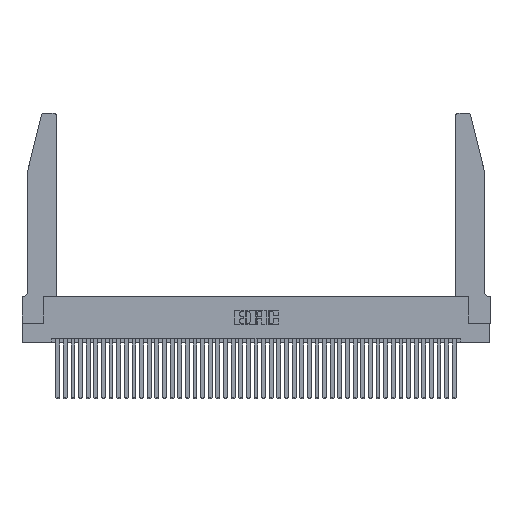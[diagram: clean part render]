
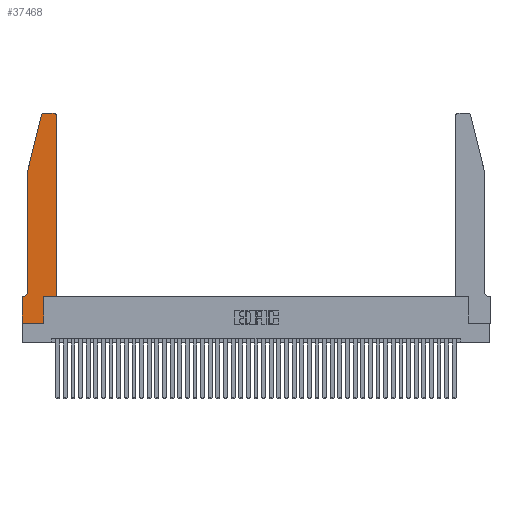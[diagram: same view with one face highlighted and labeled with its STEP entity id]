
A CAD part, top view. The second image highlights one B-rep face of the part: STEP entity #37468.
In plain terms, the highlighted planar face has unit normal (0, 0, 1).
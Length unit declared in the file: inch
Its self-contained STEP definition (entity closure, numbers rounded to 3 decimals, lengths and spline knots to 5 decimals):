
#665 = CARTESIAN_POINT ( 'NONE',  ( 0., 0., 0.37 ) ) ;
#678 = DIRECTION ( 'NONE',  ( -1., 0., 0. ) ) ;
#1070 = VERTEX_POINT ( 'NONE', #33382 ) ;
#2288 = AXIS2_PLACEMENT_3D ( 'NONE', #14128, #38184, #17613 ) ;
#2405 = DIRECTION ( 'NONE',  ( -0.239, -0.971, 0. ) ) ;
#2513 = VERTEX_POINT ( 'NONE', #38028 ) ;
#2575 = EDGE_CURVE ( 'NONE', #6158, #30357, #2855, .T. ) ;
#2855 = LINE ( 'NONE', #3952, #20219 ) ;
#3462 = CARTESIAN_POINT ( 'NONE',  ( 0.4505, 0.35, 0.37 ) ) ;
#3952 = CARTESIAN_POINT ( 'NONE',  ( 0.0755, 0.35, 0.37 ) ) ;
#4149 = VERTEX_POINT ( 'NONE', #41298 ) ;
#4229 = CARTESIAN_POINT ( 'NONE',  ( 0.0055, 0.42, 0.37 ) ) ;
#4850 = VERTEX_POINT ( 'NONE', #27520 ) ;
#4925 = AXIS2_PLACEMENT_3D ( 'NONE', #8633, #32751, #12108 ) ;
#5387 = CARTESIAN_POINT ( 'NONE',  ( 0., 0., 0.37 ) ) ;
#5448 = ORIENTED_EDGE ( 'NONE', *, *, #42419, .T. ) ;
#5553 = VECTOR ( 'NONE', #678, 39.37008 ) ;
#5979 = ORIENTED_EDGE ( 'NONE', *, *, #2575, .T. ) ;
#6158 = VERTEX_POINT ( 'NONE', #24092 ) ;
#6477 = DIRECTION ( 'NONE',  ( 0., -1., 0. ) ) ;
#6816 = AXIS2_PLACEMENT_3D ( 'NONE', #29086, #8375, #32506 ) ;
#7129 = FACE_OUTER_BOUND ( 'NONE', #15107, .T. ) ;
#7742 = DIRECTION ( 'NONE',  ( -1., 0., 0. ) ) ;
#7855 = VECTOR ( 'NONE', #44084, 39.37008 ) ;
#8115 = VECTOR ( 'NONE', #31415, 39.37008 ) ;
#8375 = DIRECTION ( 'NONE',  ( 0., 0., 1. ) ) ;
#8633 = CARTESIAN_POINT ( 'NONE',  ( 0., 0.35, 0.37 ) ) ;
#9234 = ORIENTED_EDGE ( 'NONE', *, *, #19745, .T. ) ;
#9738 = VECTOR ( 'NONE', #6477, 39.37008 ) ;
#10837 = DIRECTION ( 'NONE',  ( 0., -1., 0. ) ) ;
#10852 = EDGE_CURVE ( 'NONE', #1070, #4149, #41573, .T. ) ;
#11215 = EDGE_CURVE ( 'NONE', #37783, #1070, #34613, .T. ) ;
#11510 = EDGE_CURVE ( 'NONE', #4149, #6158, #39887, .T. ) ;
#11941 = ORIENTED_EDGE ( 'NONE', *, *, #10852, .T. ) ;
#12008 = VECTOR ( 'NONE', #10837, 39.37008 ) ;
#12108 = DIRECTION ( 'NONE',  ( 1., 0., 0. ) ) ;
#13900 = CARTESIAN_POINT ( 'NONE',  ( 0.25487, 2.72718, 0.37 ) ) ;
#14128 = CARTESIAN_POINT ( 'NONE',  ( 0.284, 2.72, 0.37 ) ) ;
#15107 = EDGE_LOOP ( 'NONE', ( #23814, #44163, #38296, #11941, #32438, #5979, #9234, #27621, #29777, #5448, #42056, #44205 ) ) ;
#15366 = VERTEX_POINT ( 'NONE', #24281 ) ;
#17125 = DIRECTION ( 'NONE',  ( 1., 0., 0. ) ) ;
#17274 = CARTESIAN_POINT ( 'NONE',  ( 0.4505, 0.35, 0.37 ) ) ;
#17304 = LINE ( 'NONE', #3462, #8115 ) ;
#17613 = DIRECTION ( 'NONE',  ( 1., 0., 0. ) ) ;
#17859 = LINE ( 'NONE', #27171, #9738 ) ;
#19745 = EDGE_CURVE ( 'NONE', #30357, #22670, #17859, .T. ) ;
#20096 = CARTESIAN_POINT ( 'NONE',  ( 0.2865, 0.35, 0.37 ) ) ;
#20219 = VECTOR ( 'NONE', #21222, 39.37008 ) ;
#21222 = DIRECTION ( 'NONE',  ( -1., 0., 0. ) ) ;
#21494 = DIRECTION ( 'NONE',  ( 1., 0., 0. ) ) ;
#21562 = VERTEX_POINT ( 'NONE', #33165 ) ;
#21604 = VERTEX_POINT ( 'NONE', #34073 ) ;
#22214 = AXIS2_PLACEMENT_3D ( 'NONE', #4229, #28439, #7742 ) ;
#22670 = VERTEX_POINT ( 'NONE', #5387 ) ;
#23056 = CARTESIAN_POINT ( 'NONE',  ( 0.0755, 2., 0.37 ) ) ;
#23814 = ORIENTED_EDGE ( 'NONE', *, *, #44483, .T. ) ;
#23932 = LINE ( 'NONE', #665, #41046 ) ;
#24092 = CARTESIAN_POINT ( 'NONE',  ( 0.0055, 0.35, 0.37 ) ) ;
#24281 = CARTESIAN_POINT ( 'NONE',  ( 0.4505, 2.72, 0.37 ) ) ;
#25860 = PLANE ( 'NONE',  #4925 ) ;
#26113 = LINE ( 'NONE', #42024, #5553 ) ;
#27034 = VERTEX_POINT ( 'NONE', #42083 ) ;
#27171 = CARTESIAN_POINT ( 'NONE',  ( 0., 0., 0.37 ) ) ;
#27520 = CARTESIAN_POINT ( 'NONE',  ( 0.2865, 0., 0.37 ) ) ;
#27621 = ORIENTED_EDGE ( 'NONE', *, *, #37291, .T. ) ;
#28223 = CIRCLE ( 'NONE', #6816, 0.03 ) ;
#28439 = DIRECTION ( 'NONE',  ( 0., 0., -1. ) ) ;
#29086 = CARTESIAN_POINT ( 'NONE',  ( 0.4205, 2.72, 0.37 ) ) ;
#29206 = CIRCLE ( 'NONE', #2288, 0.03 ) ;
#29777 = ORIENTED_EDGE ( 'NONE', *, *, #34351, .T. ) ;
#29840 = EDGE_CURVE ( 'NONE', #15366, #2513, #28223, .T. ) ;
#30357 = VERTEX_POINT ( 'NONE', #31695 ) ;
#31415 = DIRECTION ( 'NONE',  ( 0., 1., 0. ) ) ;
#31641 = EDGE_CURVE ( 'NONE', #27034, #15366, #17304, .T. ) ;
#31695 = CARTESIAN_POINT ( 'NONE',  ( 0., 0.35, 0.37 ) ) ;
#32438 = ORIENTED_EDGE ( 'NONE', *, *, #11510, .T. ) ;
#32506 = DIRECTION ( 'NONE',  ( 1., 0., 0. ) ) ;
#32751 = DIRECTION ( 'NONE',  ( 0., 0., 1. ) ) ;
#33165 = CARTESIAN_POINT ( 'NONE',  ( 0.284, 2.75, 0.37 ) ) ;
#33382 = CARTESIAN_POINT ( 'NONE',  ( 0.0755, 2., 0.37 ) ) ;
#33533 = VECTOR ( 'NONE', #2405, 39.37008 ) ;
#33817 = LINE ( 'NONE', #17274, #43959 ) ;
#34073 = CARTESIAN_POINT ( 'NONE',  ( 0.2865, 0.35, 0.37 ) ) ;
#34285 = LINE ( 'NONE', #20096, #7855 ) ;
#34351 = EDGE_CURVE ( 'NONE', #4850, #21604, #34285, .T. ) ;
#34613 = LINE ( 'NONE', #23056, #33533 ) ;
#37291 = EDGE_CURVE ( 'NONE', #22670, #4850, #23932, .T. ) ;
#37468 = ADVANCED_FACE ( 'NONE', ( #7129 ), #25860, .T. ) ;
#37783 = VERTEX_POINT ( 'NONE', #13900 ) ;
#38028 = CARTESIAN_POINT ( 'NONE',  ( 0.4205, 2.75, 0.37 ) ) ;
#38184 = DIRECTION ( 'NONE',  ( 0., 0., 1. ) ) ;
#38296 = ORIENTED_EDGE ( 'NONE', *, *, #11215, .T. ) ;
#38349 = CARTESIAN_POINT ( 'NONE',  ( 0.0755, 2., 0.37 ) ) ;
#38511 = EDGE_CURVE ( 'NONE', #21562, #37783, #29206, .T. ) ;
#39887 = CIRCLE ( 'NONE', #22214, 0.07 ) ;
#41046 = VECTOR ( 'NONE', #21494, 39.37008 ) ;
#41298 = CARTESIAN_POINT ( 'NONE',  ( 0.0755, 0.42, 0.37 ) ) ;
#41573 = LINE ( 'NONE', #38349, #12008 ) ;
#42024 = CARTESIAN_POINT ( 'NONE',  ( 0.2605, 2.75, 0.37 ) ) ;
#42056 = ORIENTED_EDGE ( 'NONE', *, *, #31641, .T. ) ;
#42083 = CARTESIAN_POINT ( 'NONE',  ( 0.4505, 0.35, 0.37 ) ) ;
#42419 = EDGE_CURVE ( 'NONE', #21604, #27034, #33817, .T. ) ;
#43959 = VECTOR ( 'NONE', #17125, 39.37008 ) ;
#44084 = DIRECTION ( 'NONE',  ( 0., 1., 0. ) ) ;
#44163 = ORIENTED_EDGE ( 'NONE', *, *, #38511, .T. ) ;
#44205 = ORIENTED_EDGE ( 'NONE', *, *, #29840, .T. ) ;
#44483 = EDGE_CURVE ( 'NONE', #2513, #21562, #26113, .T. ) ;
